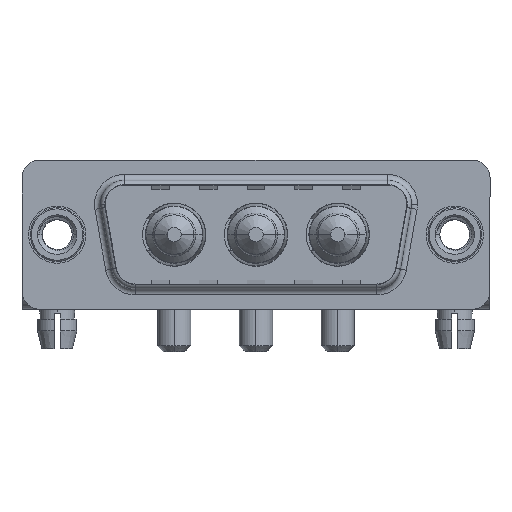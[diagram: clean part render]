
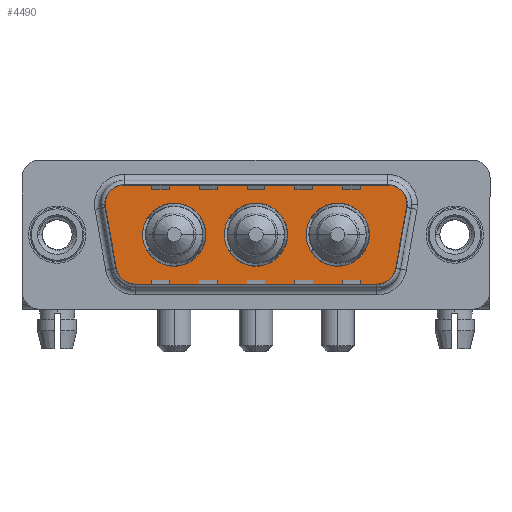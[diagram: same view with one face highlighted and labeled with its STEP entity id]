
A CAD part, top view. The second image highlights one B-rep face of the part: STEP entity #4490.
In plain terms, the highlighted planar face has unit normal (0, 0, 1).
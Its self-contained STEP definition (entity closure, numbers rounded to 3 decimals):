
#30 = DIRECTION ( 'NONE',  ( 1., 0., 0. ) ) ;
#81 = AXIS2_PLACEMENT_3D ( 'NONE', #6254, #3600, #11235 ) ;
#590 = CARTESIAN_POINT ( 'NONE',  ( 9.8, 0., 0. ) ) ;
#599 = CARTESIAN_POINT ( 'NONE',  ( 5.411, 2.9, 0. ) ) ;
#725 = CIRCLE ( 'NONE', #12803, 2. ) ;
#818 = VERTEX_POINT ( 'NONE', #12661 ) ;
#1130 = ORIENTED_EDGE ( 'NONE', *, *, #1544, .F. ) ;
#1184 = LINE ( 'NONE', #10055, #5314 ) ;
#1285 = DIRECTION ( 'NONE',  ( 0., 0., 1. ) ) ;
#1450 = CARTESIAN_POINT ( 'NONE',  ( 16.65, 0., 0. ) ) ;
#1496 = PLANE ( 'NONE',  #8768 ) ;
#1544 = EDGE_CURVE ( 'NONE', #10928, #9927, #11231, .T. ) ;
#1730 = EDGE_LOOP ( 'NONE', ( #11723, #13302, #7048, #14327, #4348, #12648, #9870, #15072, #7058 ) ) ;
#1835 = ORIENTED_EDGE ( 'NONE', *, *, #15201, .F. ) ;
#1878 = VERTEX_POINT ( 'NONE', #12328 ) ;
#2008 = DIRECTION ( 'NONE',  ( -1., 0., 0. ) ) ;
#2067 = CARTESIAN_POINT ( 'NONE',  ( 4.464, -3.247, 0. ) ) ;
#2240 = CARTESIAN_POINT ( 'NONE',  ( 5.411, 4.9, 0. ) ) ;
#2416 = EDGE_LOOP ( 'NONE', ( #3216, #1835 ) ) ;
#2426 = VERTEX_POINT ( 'NONE', #9188 ) ;
#2448 = FACE_BOUND ( 'NONE', #9453, .T. ) ;
#2552 = CARTESIAN_POINT ( 'NONE',  ( 26.15, 0., 0. ) ) ;
#2697 = ORIENTED_EDGE ( 'NONE', *, *, #9177, .F. ) ;
#2724 = LINE ( 'NONE', #14253, #5704 ) ;
#2955 = FACE_BOUND ( 'NONE', #2416, .T. ) ;
#2981 = VECTOR ( 'NONE', #6816, 1000. ) ;
#3190 = CARTESIAN_POINT ( 'NONE',  ( 19.3, 0., 0. ) ) ;
#3216 = ORIENTED_EDGE ( 'NONE', *, *, #13707, .F. ) ;
#3600 = DIRECTION ( 'NONE',  ( 0., 0., 1. ) ) ;
#3676 = AXIS2_PLACEMENT_3D ( 'NONE', #15657, #13048, #2008 ) ;
#3840 = DIRECTION ( 'NONE',  ( 0.174, 0.985, 0. ) ) ;
#3902 = CIRCLE ( 'NONE', #12397, 2. ) ;
#4222 = CIRCLE ( 'NONE', #8345, 2.65 ) ;
#4348 = ORIENTED_EDGE ( 'NONE', *, *, #4596, .T. ) ;
#4367 = DIRECTION ( 'NONE',  ( 0., 0., 1. ) ) ;
#4490 = ADVANCED_FACE ( 'NONE', ( #2448, #6238, #2955, #13264 ), #1496, .T. ) ;
#4596 = EDGE_CURVE ( 'NONE', #9503, #10946, #15783, .T. ) ;
#4749 = CIRCLE ( 'NONE', #10765, 2. ) ;
#4784 = CIRCLE ( 'NONE', #8339, 2.65 ) ;
#4856 = VERTEX_POINT ( 'NONE', #13961 ) ;
#4863 = EDGE_CURVE ( 'NONE', #9927, #10928, #6858, .T. ) ;
#5032 = CIRCLE ( 'NONE', #3676, 2. ) ;
#5056 = CARTESIAN_POINT ( 'NONE',  ( 14., 0., 0. ) ) ;
#5314 = VECTOR ( 'NONE', #6440, 1000. ) ;
#5344 = DIRECTION ( 'NONE',  ( 1., 0., 0. ) ) ;
#5400 = EDGE_CURVE ( 'NONE', #1878, #14294, #2724, .T. ) ;
#5704 = VECTOR ( 'NONE', #3840, 1000. ) ;
#5839 = DIRECTION ( 'NONE',  ( 0., 0., 1. ) ) ;
#5852 = DIRECTION ( 'NONE',  ( 1., 0., 0. ) ) ;
#5922 = CARTESIAN_POINT ( 'NONE',  ( 6.434, -2.9, 0. ) ) ;
#5941 = CARTESIAN_POINT ( 'NONE',  ( 23.5, 0., 0. ) ) ;
#6141 = EDGE_CURVE ( 'NONE', #6730, #1878, #725, .T. ) ;
#6202 = DIRECTION ( 'NONE',  ( 1., 0., 0. ) ) ;
#6238 = FACE_BOUND ( 'NONE', #6712, .T. ) ;
#6254 = CARTESIAN_POINT ( 'NONE',  ( 27.889, 2.9, 0. ) ) ;
#6418 = CIRCLE ( 'NONE', #11885, 2.65 ) ;
#6440 = DIRECTION ( 'NONE',  ( 0.174, -0.985, 0. ) ) ;
#6712 = EDGE_LOOP ( 'NONE', ( #8838, #2697 ) ) ;
#6730 = VERTEX_POINT ( 'NONE', #8033 ) ;
#6816 = DIRECTION ( 'NONE',  ( -1., 0., 0. ) ) ;
#6858 = CIRCLE ( 'NONE', #16488, 2.65 ) ;
#7048 = ORIENTED_EDGE ( 'NONE', *, *, #8415, .T. ) ;
#7058 = ORIENTED_EDGE ( 'NONE', *, *, #9170, .T. ) ;
#7328 = VERTEX_POINT ( 'NONE', #15086 ) ;
#7674 = CARTESIAN_POINT ( 'NONE',  ( 29.859, 2.553, 0. ) ) ;
#8033 = CARTESIAN_POINT ( 'NONE',  ( 26.866, -4.9, 0. ) ) ;
#8083 = DIRECTION ( 'NONE',  ( 0., 0., 1. ) ) ;
#8257 = LINE ( 'NONE', #16173, #11021 ) ;
#8339 = AXIS2_PLACEMENT_3D ( 'NONE', #10293, #15395, #12698 ) ;
#8345 = AXIS2_PLACEMENT_3D ( 'NONE', #13591, #8849, #14898 ) ;
#8415 = EDGE_CURVE ( 'NONE', #14294, #14675, #14927, .T. ) ;
#8504 = DIRECTION ( 'NONE',  ( 1., 0., 0. ) ) ;
#8768 = AXIS2_PLACEMENT_3D ( 'NONE', #14831, #14660, #30 ) ;
#8838 = ORIENTED_EDGE ( 'NONE', *, *, #12830, .F. ) ;
#8849 = DIRECTION ( 'NONE',  ( 0., 0., 1. ) ) ;
#9170 = EDGE_CURVE ( 'NONE', #2426, #6730, #8257, .T. ) ;
#9172 = EDGE_CURVE ( 'NONE', #10946, #7328, #3902, .T. ) ;
#9177 = EDGE_CURVE ( 'NONE', #12013, #9989, #14905, .T. ) ;
#9188 = CARTESIAN_POINT ( 'NONE',  ( 6.434, -4.9, 0. ) ) ;
#9453 = EDGE_LOOP ( 'NONE', ( #1130, #14997 ) ) ;
#9503 = VERTEX_POINT ( 'NONE', #12004 ) ;
#9625 = DIRECTION ( 'NONE',  ( 1., 0., 0. ) ) ;
#9694 = EDGE_CURVE ( 'NONE', #15258, #2426, #4749, .T. ) ;
#9870 = ORIENTED_EDGE ( 'NONE', *, *, #15382, .T. ) ;
#9927 = VERTEX_POINT ( 'NONE', #5056 ) ;
#9989 = VERTEX_POINT ( 'NONE', #2552 ) ;
#10055 = CARTESIAN_POINT ( 'NONE',  ( 3.441, 2.553, 0. ) ) ;
#10293 = CARTESIAN_POINT ( 'NONE',  ( 23.5, 0., 0. ) ) ;
#10765 = AXIS2_PLACEMENT_3D ( 'NONE', #5922, #4367, #15140 ) ;
#10928 = VERTEX_POINT ( 'NONE', #3190 ) ;
#10946 = VERTEX_POINT ( 'NONE', #2240 ) ;
#11021 = VECTOR ( 'NONE', #9625, 1000. ) ;
#11231 = CIRCLE ( 'NONE', #13143, 2.65 ) ;
#11235 = DIRECTION ( 'NONE',  ( -1., 0., 0. ) ) ;
#11723 = ORIENTED_EDGE ( 'NONE', *, *, #6141, .T. ) ;
#11795 = CARTESIAN_POINT ( 'NONE',  ( 20.85, 0., 0. ) ) ;
#11885 = AXIS2_PLACEMENT_3D ( 'NONE', #590, #5839, #8504 ) ;
#11926 = DIRECTION ( 'NONE',  ( 0., 0., 1. ) ) ;
#11940 = CARTESIAN_POINT ( 'NONE',  ( 26.866, -2.9, 0. ) ) ;
#12004 = CARTESIAN_POINT ( 'NONE',  ( 27.889, 4.9, 0. ) ) ;
#12013 = VERTEX_POINT ( 'NONE', #11795 ) ;
#12328 = CARTESIAN_POINT ( 'NONE',  ( 28.836, -3.247, 0. ) ) ;
#12338 = EDGE_CURVE ( 'NONE', #14675, #9503, #5032, .T. ) ;
#12367 = DIRECTION ( 'NONE',  ( 0., 0., 1. ) ) ;
#12397 = AXIS2_PLACEMENT_3D ( 'NONE', #599, #12367, #5852 ) ;
#12648 = ORIENTED_EDGE ( 'NONE', *, *, #9172, .T. ) ;
#12661 = CARTESIAN_POINT ( 'NONE',  ( 7.15, 0., 0. ) ) ;
#12698 = DIRECTION ( 'NONE',  ( 1., 0., 0. ) ) ;
#12803 = AXIS2_PLACEMENT_3D ( 'NONE', #11940, #8083, #5344 ) ;
#12830 = EDGE_CURVE ( 'NONE', #9989, #12013, #4784, .T. ) ;
#13048 = DIRECTION ( 'NONE',  ( 0., 0., 1. ) ) ;
#13143 = AXIS2_PLACEMENT_3D ( 'NONE', #16780, #1285, #6202 ) ;
#13264 = FACE_OUTER_BOUND ( 'NONE', #1730, .T. ) ;
#13302 = ORIENTED_EDGE ( 'NONE', *, *, #5400, .T. ) ;
#13591 = CARTESIAN_POINT ( 'NONE',  ( 9.8, 0., 0. ) ) ;
#13707 = EDGE_CURVE ( 'NONE', #4856, #818, #4222, .T. ) ;
#13856 = DIRECTION ( 'NONE',  ( 1., 0., 0. ) ) ;
#13961 = CARTESIAN_POINT ( 'NONE',  ( 12.45, 0., 0. ) ) ;
#14253 = CARTESIAN_POINT ( 'NONE',  ( 29.859, 2.553, 0. ) ) ;
#14294 = VERTEX_POINT ( 'NONE', #7674 ) ;
#14327 = ORIENTED_EDGE ( 'NONE', *, *, #12338, .T. ) ;
#14343 = AXIS2_PLACEMENT_3D ( 'NONE', #5941, #16437, #13856 ) ;
#14660 = DIRECTION ( 'NONE',  ( 0., 0., 1. ) ) ;
#14675 = VERTEX_POINT ( 'NONE', #15257 ) ;
#14831 = CARTESIAN_POINT ( 'NONE',  ( 26.866, -2.9, 0. ) ) ;
#14898 = DIRECTION ( 'NONE',  ( 1., 0., 0. ) ) ;
#14905 = CIRCLE ( 'NONE', #14343, 2.65 ) ;
#14927 = CIRCLE ( 'NONE', #81, 2. ) ;
#14997 = ORIENTED_EDGE ( 'NONE', *, *, #4863, .F. ) ;
#15072 = ORIENTED_EDGE ( 'NONE', *, *, #9694, .T. ) ;
#15086 = CARTESIAN_POINT ( 'NONE',  ( 3.441, 2.553, 0. ) ) ;
#15140 = DIRECTION ( 'NONE',  ( -1., 0., 0. ) ) ;
#15201 = EDGE_CURVE ( 'NONE', #818, #4856, #6418, .T. ) ;
#15257 = CARTESIAN_POINT ( 'NONE',  ( 29.889, 2.9, 0. ) ) ;
#15258 = VERTEX_POINT ( 'NONE', #2067 ) ;
#15382 = EDGE_CURVE ( 'NONE', #7328, #15258, #1184, .T. ) ;
#15395 = DIRECTION ( 'NONE',  ( 0., 0., 1. ) ) ;
#15657 = CARTESIAN_POINT ( 'NONE',  ( 27.889, 2.9, 0. ) ) ;
#15783 = LINE ( 'NONE', #15942, #2981 ) ;
#15905 = DIRECTION ( 'NONE',  ( 1., 0., 0. ) ) ;
#15942 = CARTESIAN_POINT ( 'NONE',  ( 5.411, 4.9, 0. ) ) ;
#16173 = CARTESIAN_POINT ( 'NONE',  ( 6.434, -4.9, 0. ) ) ;
#16437 = DIRECTION ( 'NONE',  ( 0., 0., 1. ) ) ;
#16488 = AXIS2_PLACEMENT_3D ( 'NONE', #1450, #11926, #15905 ) ;
#16780 = CARTESIAN_POINT ( 'NONE',  ( 16.65, 0., 0. ) ) ;
